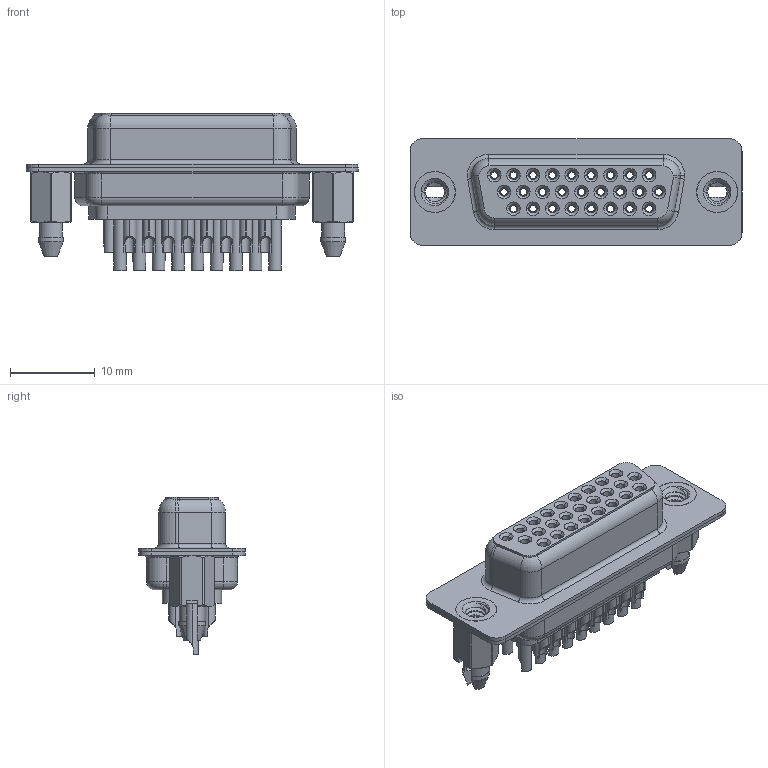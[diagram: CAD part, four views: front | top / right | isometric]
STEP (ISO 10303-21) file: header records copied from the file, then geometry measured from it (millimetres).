
FILE_DESCRIPTION (( 'STEP AP203' ), '1' );
FILE_NAME ('638-026-632-266.STEP', '2020-07-18T21:56:42', ( '' ), ( '' ), 'SwSTEP 2.0', 'SolidWorks 2020', '' );
FILE_SCHEMA (( 'CONFIG_CONTROL_DESIGN' ));
Length unit declared in the file: millimetre
Products named in the file (8): 638 Contact Row 3_32; 638 Housing_26 Contacts; 638-026-632-266; 638 Contact Row 2_32; 638 Contact Row 1_32; 638 4-40 Threaded Boardlock_LP; 638 Shell Front_26 Contacts; 638 Shell Rear_26 Contacts
Assembly tree (31 placements, depth 2):
  638-026-632-266
    638 Housing_26 Contacts
    638 Shell Front_26 Contacts
    638 Shell Rear_26 Contacts
    638 Contact Row 1_32  x9
    638 Contact Row 2_32  x9
    638 Contact Row 3_32  x8
    638 4-40 Threaded Boardlock_LP  x2
Bounding box: 39.19 x 12.6 x 18.6 mm (x, y, z)
Volume: 2374.2 mm3; surface area: 9053.6 mm2
Topology: 31 solids, 31 shells, 2667 faces, 6793 edges, 4275 vertices
Faces by surface type: cylinder 819, plane 645, bspline 526, torus 525, cone 152
Entity records: 30019 total; most frequent: CARTESIAN_POINT 8653, DIRECTION 4298, ORIENTED_EDGE 4084, EDGE_CURVE 2042, AXIS2_PLACEMENT_3D 1787, VERTEX_POINT 1293, EDGE_LOOP 1001, CIRCLE 967
